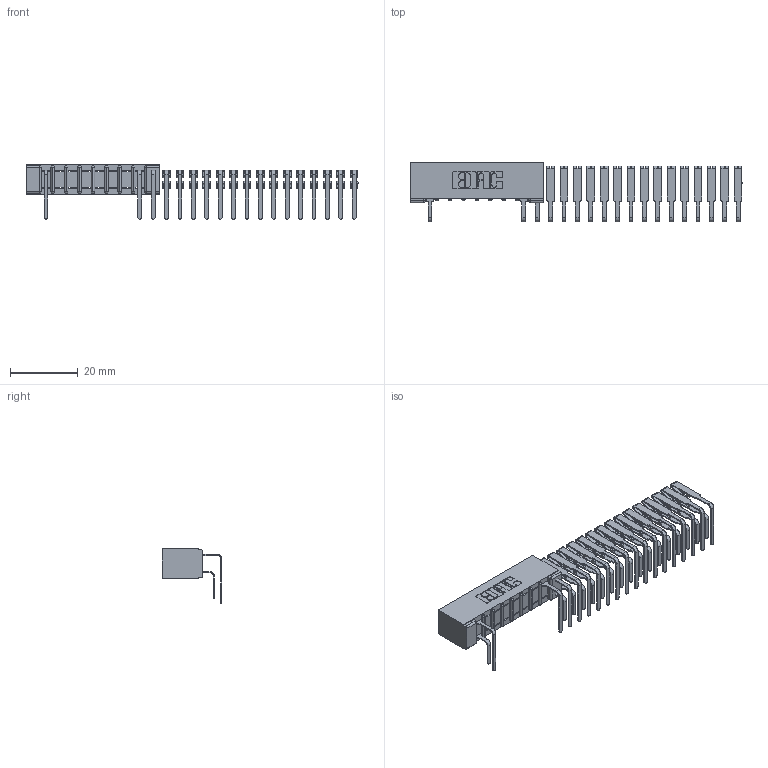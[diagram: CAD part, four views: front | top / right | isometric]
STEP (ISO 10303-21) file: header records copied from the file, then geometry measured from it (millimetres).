
FILE_DESCRIPTION (( 'STEP AP203' ), '1' );
FILE_NAME ('357-024-559-101.STEP', '2018-08-09T00:22:18', ( '' ), ( '' ), 'SwSTEP 2.0', 'SolidWorks 2016', '' );
FILE_SCHEMA (( 'CONFIG_CONTROL_DESIGN' ));
Length unit declared in the file: inch
Products named in the file (4): 357-024-559-101; 307 Part_No Mounting Lugs; 307-290-001_558 559 - 1 (Single); 307-290-001_559 - 2 (Single)
Assembly tree (36 placements, depth 2):
  357-024-559-101
    307 Part_No Mounting Lugs
    307-290-001_558 559 - 1 (Single)  x17
    307-290-001_559 - 2 (Single)  x18
Bounding box: 98.18 x 17.69 x 16.08 mm (x, y, z)
Volume: 3226 mm3; surface area: 7774.7 mm2
Topology: 36 solids, 36 shells, 1679 faces, 4661 edges, 3034 vertices
Faces by surface type: plane 1107, cylinder 554, sphere 18
Entity records: 13083 total; most frequent: CARTESIAN_POINT 2069, DIRECTION 2059, ORIENTED_EDGE 2026, EDGE_CURVE 1013, VECTOR 763, LINE 763, VERTEX_POINT 658, AXIS2_PLACEMENT_3D 648
